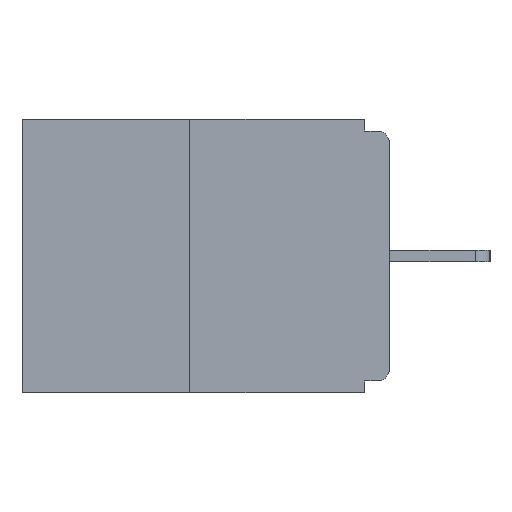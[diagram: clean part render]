
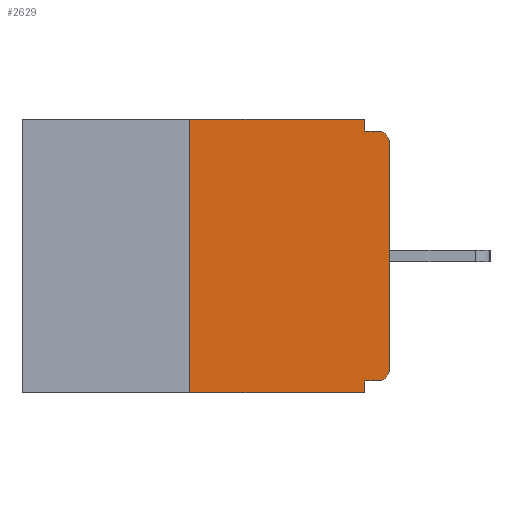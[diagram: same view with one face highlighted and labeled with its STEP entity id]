
A CAD part, left-side view. The second image highlights one B-rep face of the part: STEP entity #2629.
In plain terms, the highlighted planar face has unit normal (-1, 0, 0).
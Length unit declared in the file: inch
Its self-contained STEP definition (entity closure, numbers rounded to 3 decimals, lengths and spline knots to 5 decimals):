
#316 = VECTOR ( 'NONE', #1104, 39.37008 ) ;
#339 = EDGE_CURVE ( 'NONE', #21641, #15450, #13750, .T. ) ;
#547 = ORIENTED_EDGE ( 'NONE', *, *, #8903, .F. ) ;
#1104 = DIRECTION ( 'NONE',  ( 0., 0., -1. ) ) ;
#1319 = DIRECTION ( 'NONE',  ( 1., 0., 0. ) ) ;
#1480 = CARTESIAN_POINT ( 'NONE',  ( 0., 0.25, 0. ) ) ;
#2047 = EDGE_LOOP ( 'NONE', ( #25034, #547, #25090, #25176, #8142, #22480, #20525, #19232, #19820, #15668 ) ) ;
#2166 = CARTESIAN_POINT ( 'NONE',  ( 0., 0.031, -0.343 ) ) ;
#2629 = ADVANCED_FACE ( 'NONE', ( #23479 ), #5691, .F. ) ;
#2698 = VERTEX_POINT ( 'NONE', #21133 ) ;
#2969 = DIRECTION ( 'NONE',  ( -1., 0., 0. ) ) ;
#3059 = CARTESIAN_POINT ( 'NONE',  ( 0., 0.015, -0.313 ) ) ;
#3245 = CARTESIAN_POINT ( 'NONE',  ( 0., 0., -0.03 ) ) ;
#3469 = LINE ( 'NONE', #11459, #8015 ) ;
#3737 = VERTEX_POINT ( 'NONE', #13201 ) ;
#3775 = EDGE_CURVE ( 'NONE', #24065, #9447, #17286, .T. ) ;
#3798 = VECTOR ( 'NONE', #3980, 39.37008 ) ;
#3980 = DIRECTION ( 'NONE',  ( 0., 0., -1. ) ) ;
#4835 = DIRECTION ( 'NONE',  ( 0., -1., 0. ) ) ;
#4866 = DIRECTION ( 'NONE',  ( -1., 0., 0. ) ) ;
#4983 = CARTESIAN_POINT ( 'NONE',  ( 0., 0.25, -0.343 ) ) ;
#5033 = AXIS2_PLACEMENT_3D ( 'NONE', #5569, #1319, #9716 ) ;
#5569 = CARTESIAN_POINT ( 'NONE',  ( 0., 0.46, 0. ) ) ;
#5691 = PLANE ( 'NONE',  #5033 ) ;
#6318 = CARTESIAN_POINT ( 'NONE',  ( 0., 0.031, -0.328 ) ) ;
#6685 = EDGE_CURVE ( 'NONE', #18899, #23111, #11545, .T. ) ;
#7010 = LINE ( 'NONE', #1480, #16382 ) ;
#8015 = VECTOR ( 'NONE', #9277, 39.37008 ) ;
#8142 = ORIENTED_EDGE ( 'NONE', *, *, #21148, .F. ) ;
#8433 = DIRECTION ( 'NONE',  ( 0., -1., 0. ) ) ;
#8766 = EDGE_CURVE ( 'NONE', #9447, #2698, #12293, .T. ) ;
#8903 = EDGE_CURVE ( 'NONE', #17463, #3737, #7010, .T. ) ;
#9114 = DIRECTION ( 'NONE',  ( 0., 0., -1. ) ) ;
#9277 = DIRECTION ( 'NONE',  ( 0., 1., 0. ) ) ;
#9410 = CARTESIAN_POINT ( 'NONE',  ( 0., 0.031, -0.343 ) ) ;
#9447 = VERTEX_POINT ( 'NONE', #14081 ) ;
#9604 = CIRCLE ( 'NONE', #19000, 0.015 ) ;
#9716 = DIRECTION ( 'NONE',  ( 0., 0., -1. ) ) ;
#10712 = CARTESIAN_POINT ( 'NONE',  ( 0., 0.015, -0.03 ) ) ;
#10901 = LINE ( 'NONE', #12941, #22796 ) ;
#11091 = EDGE_CURVE ( 'NONE', #17266, #18899, #21050, .T. ) ;
#11302 = DIRECTION ( 'NONE',  ( 0., 0., 1. ) ) ;
#11459 = CARTESIAN_POINT ( 'NONE',  ( 0., 0., -0.328 ) ) ;
#11545 = LINE ( 'NONE', #25332, #15960 ) ;
#12223 = LINE ( 'NONE', #12471, #19344 ) ;
#12293 = LINE ( 'NONE', #24257, #24625 ) ;
#12471 = CARTESIAN_POINT ( 'NONE',  ( 0., 0.46, -0.343 ) ) ;
#12630 = DIRECTION ( 'NONE',  ( 0., 0., -1. ) ) ;
#12662 = EDGE_CURVE ( 'NONE', #3737, #24065, #10901, .T. ) ;
#12941 = CARTESIAN_POINT ( 'NONE',  ( 0., 0.46, 0. ) ) ;
#13201 = CARTESIAN_POINT ( 'NONE',  ( 0., 0.25, 0. ) ) ;
#13750 = LINE ( 'NONE', #9410, #3798 ) ;
#14059 = AXIS2_PLACEMENT_3D ( 'NONE', #3059, #4866, #9114 ) ;
#14081 = CARTESIAN_POINT ( 'NONE',  ( 0., 0.031, -0.015 ) ) ;
#14373 = DIRECTION ( 'NONE',  ( 0., -1., 0. ) ) ;
#14977 = DIRECTION ( 'NONE',  ( 0., 0., 1. ) ) ;
#15450 = VERTEX_POINT ( 'NONE', #2166 ) ;
#15668 = ORIENTED_EDGE ( 'NONE', *, *, #3775, .F. ) ;
#15960 = VECTOR ( 'NONE', #11302, 39.37008 ) ;
#16382 = VECTOR ( 'NONE', #14977, 39.37008 ) ;
#16399 = CARTESIAN_POINT ( 'NONE',  ( 0., 0.015, -0.328 ) ) ;
#17170 = CARTESIAN_POINT ( 'NONE',  ( 0., 0.031, 0. ) ) ;
#17266 = VERTEX_POINT ( 'NONE', #16399 ) ;
#17286 = LINE ( 'NONE', #17170, #316 ) ;
#17398 = CARTESIAN_POINT ( 'NONE',  ( 0., 0.031, 0. ) ) ;
#17463 = VERTEX_POINT ( 'NONE', #4983 ) ;
#17702 = CARTESIAN_POINT ( 'NONE',  ( 0., 0., -0.313 ) ) ;
#18215 = EDGE_CURVE ( 'NONE', #23111, #2698, #9604, .T. ) ;
#18899 = VERTEX_POINT ( 'NONE', #17702 ) ;
#19000 = AXIS2_PLACEMENT_3D ( 'NONE', #10712, #2969, #12630 ) ;
#19232 = ORIENTED_EDGE ( 'NONE', *, *, #18215, .T. ) ;
#19344 = VECTOR ( 'NONE', #14373, 39.37008 ) ;
#19820 = ORIENTED_EDGE ( 'NONE', *, *, #8766, .F. ) ;
#20525 = ORIENTED_EDGE ( 'NONE', *, *, #6685, .T. ) ;
#21050 = CIRCLE ( 'NONE', #14059, 0.015 ) ;
#21133 = CARTESIAN_POINT ( 'NONE',  ( 0., 0.015, -0.015 ) ) ;
#21148 = EDGE_CURVE ( 'NONE', #17266, #21641, #3469, .T. ) ;
#21641 = VERTEX_POINT ( 'NONE', #6318 ) ;
#22082 = EDGE_CURVE ( 'NONE', #17463, #15450, #12223, .T. ) ;
#22480 = ORIENTED_EDGE ( 'NONE', *, *, #11091, .T. ) ;
#22796 = VECTOR ( 'NONE', #4835, 39.37008 ) ;
#23111 = VERTEX_POINT ( 'NONE', #3245 ) ;
#23479 = FACE_OUTER_BOUND ( 'NONE', #2047, .T. ) ;
#24065 = VERTEX_POINT ( 'NONE', #17398 ) ;
#24257 = CARTESIAN_POINT ( 'NONE',  ( 0., 0., -0.015 ) ) ;
#24625 = VECTOR ( 'NONE', #8433, 39.37008 ) ;
#25034 = ORIENTED_EDGE ( 'NONE', *, *, #12662, .F. ) ;
#25090 = ORIENTED_EDGE ( 'NONE', *, *, #22082, .T. ) ;
#25176 = ORIENTED_EDGE ( 'NONE', *, *, #339, .F. ) ;
#25332 = CARTESIAN_POINT ( 'NONE',  ( 0., 0., 0. ) ) ;
